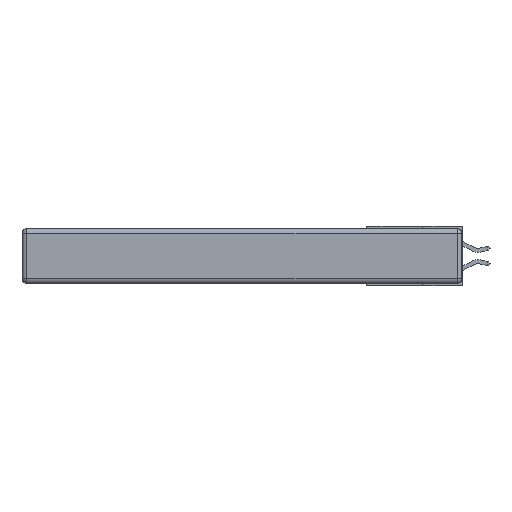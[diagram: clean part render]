
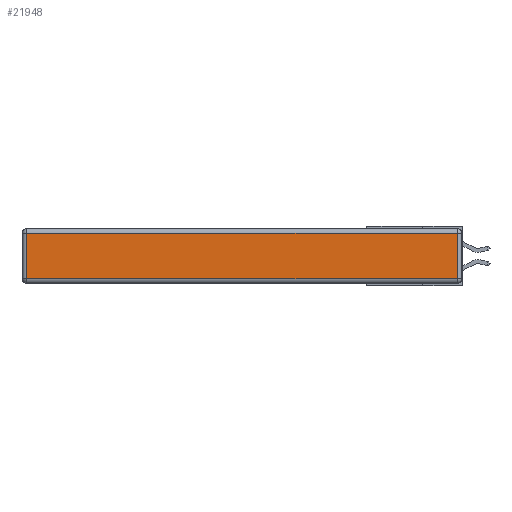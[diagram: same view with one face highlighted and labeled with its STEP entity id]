
A CAD part, left-side view. The second image highlights one B-rep face of the part: STEP entity #21948.
In plain terms, the highlighted planar face has unit normal (-1, 0, 0).
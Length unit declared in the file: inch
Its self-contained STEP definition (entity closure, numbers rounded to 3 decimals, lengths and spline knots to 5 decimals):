
#613 = DIRECTION ( 'NONE',  ( 0., -1., 0. ) ) ;
#718 = FACE_OUTER_BOUND ( 'NONE', #9949, .T. ) ;
#1428 = CARTESIAN_POINT ( 'NONE',  ( 0., 2.72, -0.03 ) ) ;
#1897 = VECTOR ( 'NONE', #27379, 39.37008 ) ;
#2046 = ORIENTED_EDGE ( 'NONE', *, *, #19552, .T. ) ;
#3930 = DIRECTION ( 'NONE',  ( 0., 1., 0. ) ) ;
#4030 = CARTESIAN_POINT ( 'NONE',  ( 0., 0., -0.343 ) ) ;
#5086 = VECTOR ( 'NONE', #3930, 39.37008 ) ;
#5643 = AXIS2_PLACEMENT_3D ( 'NONE', #4030, #17269, #19060 ) ;
#7407 = VERTEX_POINT ( 'NONE', #22811 ) ;
#8375 = LINE ( 'NONE', #10552, #5086 ) ;
#8971 = ORIENTED_EDGE ( 'NONE', *, *, #27676, .T. ) ;
#9949 = EDGE_LOOP ( 'NONE', ( #2046, #8971, #16423, #18997 ) ) ;
#10552 = CARTESIAN_POINT ( 'NONE',  ( 0., 2.75, -0.03 ) ) ;
#13140 = VECTOR ( 'NONE', #26830, 39.37008 ) ;
#13538 = EDGE_CURVE ( 'NONE', #18495, #16085, #22248, .T. ) ;
#14376 = EDGE_CURVE ( 'NONE', #7407, #18495, #8375, .T. ) ;
#16085 = VERTEX_POINT ( 'NONE', #24989 ) ;
#16423 = ORIENTED_EDGE ( 'NONE', *, *, #14376, .T. ) ;
#16623 = LINE ( 'NONE', #27473, #1897 ) ;
#16887 = CARTESIAN_POINT ( 'NONE',  ( 0., 0.03, -0.313 ) ) ;
#17269 = DIRECTION ( 'NONE',  ( -1., 0., 0. ) ) ;
#17472 = CARTESIAN_POINT ( 'NONE',  ( 0., 0., -0.313 ) ) ;
#18291 = LINE ( 'NONE', #17472, #26034 ) ;
#18495 = VERTEX_POINT ( 'NONE', #1428 ) ;
#18997 = ORIENTED_EDGE ( 'NONE', *, *, #13538, .T. ) ;
#19060 = DIRECTION ( 'NONE',  ( 0., 0., 1. ) ) ;
#19552 = EDGE_CURVE ( 'NONE', #16085, #26882, #18291, .T. ) ;
#21948 = ADVANCED_FACE ( 'NONE', ( #718 ), #27627, .T. ) ;
#22248 = LINE ( 'NONE', #25117, #13140 ) ;
#22811 = CARTESIAN_POINT ( 'NONE',  ( 0., 0.03, -0.03 ) ) ;
#24989 = CARTESIAN_POINT ( 'NONE',  ( 0., 2.72, -0.313 ) ) ;
#25117 = CARTESIAN_POINT ( 'NONE',  ( 0., 2.72, -0.343 ) ) ;
#26034 = VECTOR ( 'NONE', #613, 39.37008 ) ;
#26830 = DIRECTION ( 'NONE',  ( 0., 0., -1. ) ) ;
#26882 = VERTEX_POINT ( 'NONE', #16887 ) ;
#27379 = DIRECTION ( 'NONE',  ( 0., 0., 1. ) ) ;
#27473 = CARTESIAN_POINT ( 'NONE',  ( 0., 0.03, -0.343 ) ) ;
#27627 = PLANE ( 'NONE',  #5643 ) ;
#27676 = EDGE_CURVE ( 'NONE', #26882, #7407, #16623, .T. ) ;
